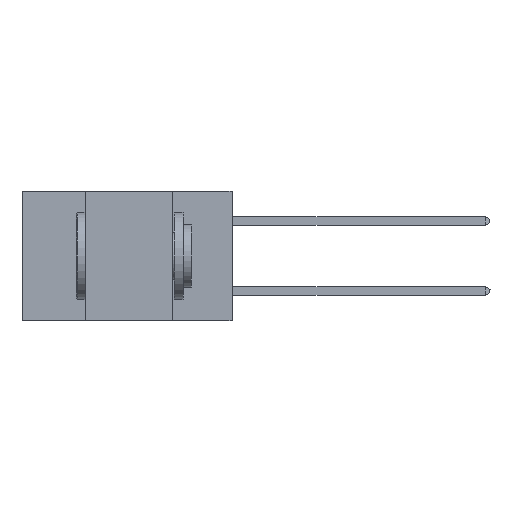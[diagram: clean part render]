
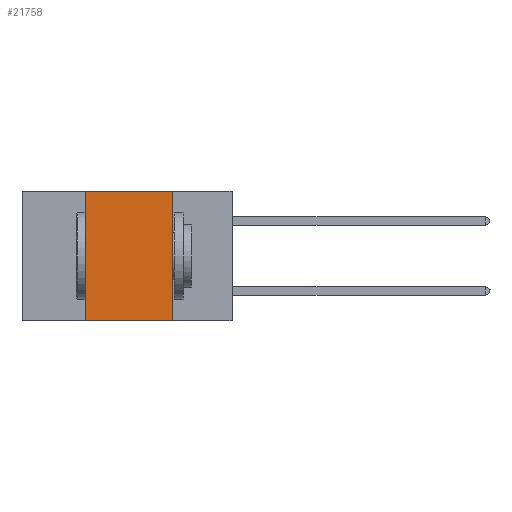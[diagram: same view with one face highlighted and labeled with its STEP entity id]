
A CAD part, left-side view. The second image highlights one B-rep face of the part: STEP entity #21758.
In plain terms, the highlighted planar face has unit normal (-1, 0, 0).
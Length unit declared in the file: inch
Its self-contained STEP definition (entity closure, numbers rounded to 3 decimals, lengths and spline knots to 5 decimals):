
#96 = ORIENTED_EDGE ( 'NONE', *, *, #18950, .F. ) ;
#668 = DIRECTION ( 'NONE',  ( 0., 0., -1. ) ) ;
#804 = DIRECTION ( 'NONE',  ( 0., -1., 0. ) ) ;
#2914 = DIRECTION ( 'NONE',  ( 0., -1., 0. ) ) ;
#3059 = EDGE_LOOP ( 'NONE', ( #12589, #25152, #96, #23897 ) ) ;
#3273 = CARTESIAN_POINT ( 'NONE',  ( 0., 0.6, 0. ) ) ;
#4461 = LINE ( 'NONE', #30364, #17339 ) ;
#4468 = CARTESIAN_POINT ( 'NONE',  ( 0., 0.17, 0. ) ) ;
#5547 = EDGE_CURVE ( 'NONE', #30005, #17718, #30483, .T. ) ;
#5663 = DIRECTION ( 'NONE',  ( 0., 0., -1. ) ) ;
#6118 = DIRECTION ( 'NONE',  ( 0., 0., 1. ) ) ;
#10719 = VECTOR ( 'NONE', #6118, 39.37008 ) ;
#12364 = LINE ( 'NONE', #18922, #10719 ) ;
#12589 = ORIENTED_EDGE ( 'NONE', *, *, #24196, .F. ) ;
#12986 = EDGE_CURVE ( 'NONE', #21160, #30454, #4461, .T. ) ;
#13828 = AXIS2_PLACEMENT_3D ( 'NONE', #3273, #30600, #5663 ) ;
#15623 = FACE_OUTER_BOUND ( 'NONE', #3059, .T. ) ;
#15854 = VECTOR ( 'NONE', #2914, 39.37008 ) ;
#17320 = CARTESIAN_POINT ( 'NONE',  ( 0., 0.17, 0. ) ) ;
#17339 = VECTOR ( 'NONE', #804, 39.37008 ) ;
#17420 = CARTESIAN_POINT ( 'NONE',  ( 0., 0.42, 0. ) ) ;
#17718 = VERTEX_POINT ( 'NONE', #27266 ) ;
#17970 = CARTESIAN_POINT ( 'NONE',  ( 0., 0.42, -0.37 ) ) ;
#18047 = CARTESIAN_POINT ( 'NONE',  ( 0., 0.6, -0.37 ) ) ;
#18922 = CARTESIAN_POINT ( 'NONE',  ( 0., 0.42, 0. ) ) ;
#18950 = EDGE_CURVE ( 'NONE', #30005, #21160, #12364, .T. ) ;
#21160 = VERTEX_POINT ( 'NONE', #17420 ) ;
#21758 = ADVANCED_FACE ( 'NONE', ( #15623 ), #23322, .F. ) ;
#23322 = PLANE ( 'NONE',  #13828 ) ;
#23897 = ORIENTED_EDGE ( 'NONE', *, *, #5547, .T. ) ;
#24196 = EDGE_CURVE ( 'NONE', #30454, #17718, #32308, .T. ) ;
#25152 = ORIENTED_EDGE ( 'NONE', *, *, #12986, .F. ) ;
#25606 = VECTOR ( 'NONE', #668, 39.37008 ) ;
#27266 = CARTESIAN_POINT ( 'NONE',  ( 0., 0.17, -0.37 ) ) ;
#30005 = VERTEX_POINT ( 'NONE', #17970 ) ;
#30364 = CARTESIAN_POINT ( 'NONE',  ( 0., 0.6, 0. ) ) ;
#30454 = VERTEX_POINT ( 'NONE', #4468 ) ;
#30483 = LINE ( 'NONE', #18047, #15854 ) ;
#30600 = DIRECTION ( 'NONE',  ( 1., 0., 0. ) ) ;
#32308 = LINE ( 'NONE', #17320, #25606 ) ;
